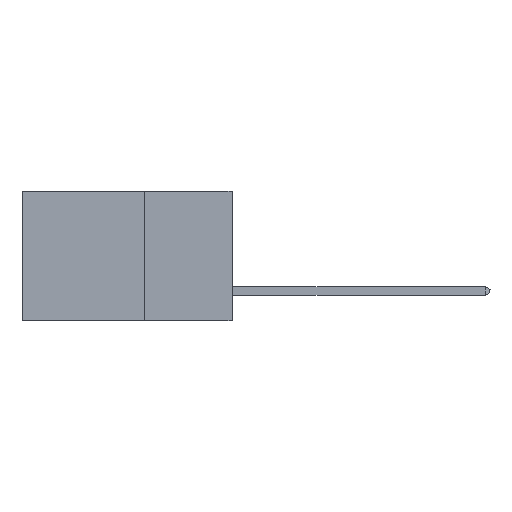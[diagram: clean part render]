
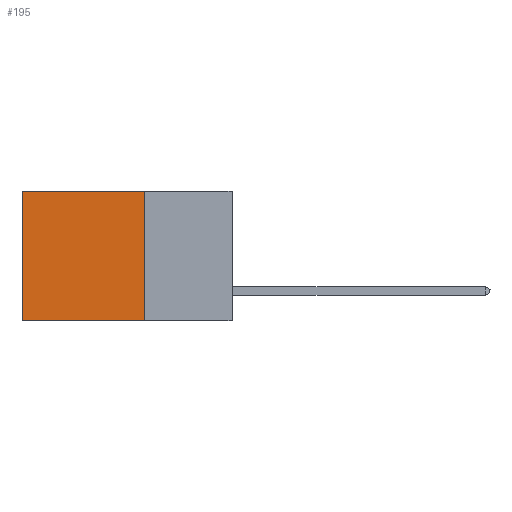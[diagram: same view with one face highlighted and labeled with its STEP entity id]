
A CAD part, left-side view. The second image highlights one B-rep face of the part: STEP entity #195.
In plain terms, the highlighted planar face has unit normal (-1, 0, 0).
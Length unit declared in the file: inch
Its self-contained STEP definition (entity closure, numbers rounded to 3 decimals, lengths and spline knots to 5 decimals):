
#195 = ADVANCED_FACE ( 'NONE', ( #8696 ), #23152, .F. ) ;
#1085 = ORIENTED_EDGE ( 'NONE', *, *, #24826, .F. ) ;
#1922 = ORIENTED_EDGE ( 'NONE', *, *, #5080, .F. ) ;
#1978 = ORIENTED_EDGE ( 'NONE', *, *, #5168, .T. ) ;
#2304 = LINE ( 'NONE', #18433, #22400 ) ;
#2573 = VECTOR ( 'NONE', #23006, 39.37008 ) ;
#2736 = CARTESIAN_POINT ( 'NONE',  ( 0.2875, 0.6, 0. ) ) ;
#3780 = CARTESIAN_POINT ( 'NONE',  ( 0.2875, 0.25, 0. ) ) ;
#4232 = CARTESIAN_POINT ( 'NONE',  ( 0.2875, 0.6, 0. ) ) ;
#4408 = LINE ( 'NONE', #6464, #2573 ) ;
#4702 = DIRECTION ( 'NONE',  ( 0., 0., -1. ) ) ;
#5080 = EDGE_CURVE ( 'NONE', #15156, #21041, #4408, .T. ) ;
#5168 = EDGE_CURVE ( 'NONE', #15440, #21041, #14796, .T. ) ;
#6464 = CARTESIAN_POINT ( 'NONE',  ( 0.2875, 0.25, -0.37 ) ) ;
#8696 = FACE_OUTER_BOUND ( 'NONE', #27104, .T. ) ;
#8842 = VECTOR ( 'NONE', #26583, 39.37008 ) ;
#10120 = CARTESIAN_POINT ( 'NONE',  ( 0.2875, 0.25, -0.37 ) ) ;
#13617 = ORIENTED_EDGE ( 'NONE', *, *, #23884, .T. ) ;
#13930 = DIRECTION ( 'NONE',  ( 1., 0., 0. ) ) ;
#13987 = CARTESIAN_POINT ( 'NONE',  ( 0.2875, 0.25, 0. ) ) ;
#14317 = AXIS2_PLACEMENT_3D ( 'NONE', #25743, #13930, #25645 ) ;
#14796 = LINE ( 'NONE', #4232, #15143 ) ;
#15143 = VECTOR ( 'NONE', #29533, 39.37008 ) ;
#15156 = VERTEX_POINT ( 'NONE', #10120 ) ;
#15440 = VERTEX_POINT ( 'NONE', #2736 ) ;
#18433 = CARTESIAN_POINT ( 'NONE',  ( 0.2875, 0.25, 0. ) ) ;
#20874 = CARTESIAN_POINT ( 'NONE',  ( 0.2875, 0.6, -0.37 ) ) ;
#21041 = VERTEX_POINT ( 'NONE', #20874 ) ;
#22400 = VECTOR ( 'NONE', #4702, 39.37008 ) ;
#23006 = DIRECTION ( 'NONE',  ( 0., 1., 0. ) ) ;
#23142 = VERTEX_POINT ( 'NONE', #13987 ) ;
#23152 = PLANE ( 'NONE',  #14317 ) ;
#23884 = EDGE_CURVE ( 'NONE', #23142, #15440, #27178, .T. ) ;
#24826 = EDGE_CURVE ( 'NONE', #23142, #15156, #2304, .T. ) ;
#25645 = DIRECTION ( 'NONE',  ( 0., 0., -1. ) ) ;
#25743 = CARTESIAN_POINT ( 'NONE',  ( 0.2875, 0.25, 0. ) ) ;
#26583 = DIRECTION ( 'NONE',  ( 0., 1., 0. ) ) ;
#27104 = EDGE_LOOP ( 'NONE', ( #1978, #1922, #1085, #13617 ) ) ;
#27178 = LINE ( 'NONE', #3780, #8842 ) ;
#29533 = DIRECTION ( 'NONE',  ( 0., 0., -1. ) ) ;
